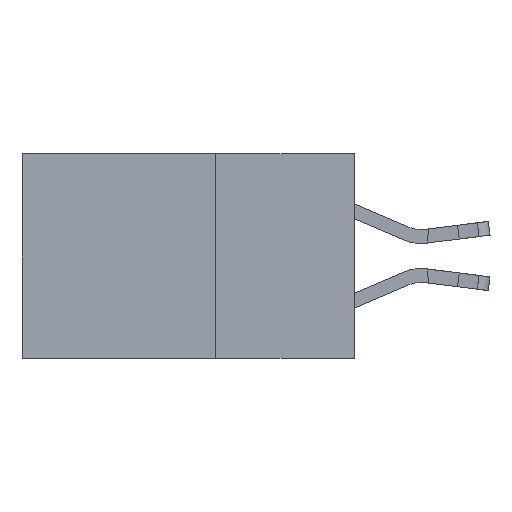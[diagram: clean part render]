
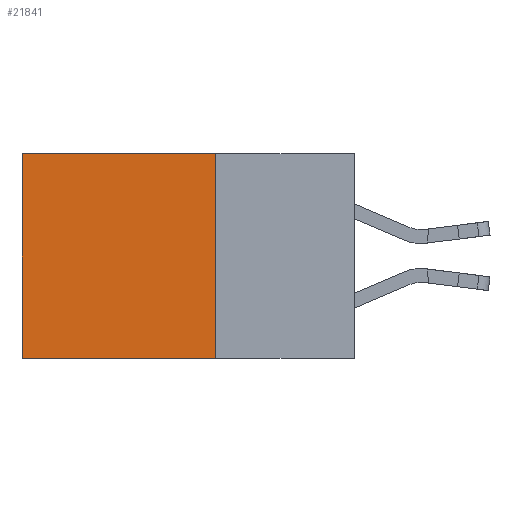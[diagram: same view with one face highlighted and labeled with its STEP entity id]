
A CAD part, left-side view. The second image highlights one B-rep face of the part: STEP entity #21841.
In plain terms, the highlighted planar face has unit normal (-1, 0, 0).
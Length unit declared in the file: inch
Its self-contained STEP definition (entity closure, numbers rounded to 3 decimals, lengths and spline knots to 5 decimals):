
#65 = LINE ( 'NONE', #18671, #18325 ) ;
#233 = LINE ( 'NONE', #8645, #21124 ) ;
#1150 = CARTESIAN_POINT ( 'NONE',  ( 0.2615, 0.25, 0. ) ) ;
#2202 = DIRECTION ( 'NONE',  ( 0., 0., -1. ) ) ;
#2659 = CARTESIAN_POINT ( 'NONE',  ( 0.2615, 0.6, -0.37 ) ) ;
#3475 = EDGE_CURVE ( 'NONE', #10240, #20076, #233, .T. ) ;
#3561 = ORIENTED_EDGE ( 'NONE', *, *, #3475, .F. ) ;
#3818 = VERTEX_POINT ( 'NONE', #10175 ) ;
#3977 = EDGE_CURVE ( 'NONE', #10240, #3818, #4320, .T. ) ;
#4320 = LINE ( 'NONE', #1150, #20062 ) ;
#6410 = DIRECTION ( 'NONE',  ( 1., 0., 0. ) ) ;
#7657 = AXIS2_PLACEMENT_3D ( 'NONE', #21619, #6410, #19941 ) ;
#8099 = FACE_OUTER_BOUND ( 'NONE', #13584, .T. ) ;
#8645 = CARTESIAN_POINT ( 'NONE',  ( 0.2615, 0.25, -0.37 ) ) ;
#9176 = ORIENTED_EDGE ( 'NONE', *, *, #10137, .F. ) ;
#9628 = ORIENTED_EDGE ( 'NONE', *, *, #3977, .T. ) ;
#10137 = EDGE_CURVE ( 'NONE', #20076, #20198, #65, .T. ) ;
#10175 = CARTESIAN_POINT ( 'NONE',  ( 0.2615, 0.6, 0. ) ) ;
#10240 = VERTEX_POINT ( 'NONE', #15453 ) ;
#10302 = ORIENTED_EDGE ( 'NONE', *, *, #20506, .T. ) ;
#12171 = CARTESIAN_POINT ( 'NONE',  ( 0.2615, 0.6, -0.37 ) ) ;
#13584 = EDGE_LOOP ( 'NONE', ( #10302, #9176, #3561, #9628 ) ) ;
#13974 = CARTESIAN_POINT ( 'NONE',  ( 0.2615, 0.25, -0.37 ) ) ;
#14558 = DIRECTION ( 'NONE',  ( 0., 1., 0. ) ) ;
#14868 = PLANE ( 'NONE',  #7657 ) ;
#15412 = DIRECTION ( 'NONE',  ( 0., 0., -1. ) ) ;
#15453 = CARTESIAN_POINT ( 'NONE',  ( 0.2615, 0.25, 0. ) ) ;
#16698 = DIRECTION ( 'NONE',  ( 0., 1., 0. ) ) ;
#17503 = VECTOR ( 'NONE', #2202, 39.37008 ) ;
#18325 = VECTOR ( 'NONE', #16698, 39.37008 ) ;
#18671 = CARTESIAN_POINT ( 'NONE',  ( 0.2615, 0.25, -0.37 ) ) ;
#18724 = LINE ( 'NONE', #12171, #17503 ) ;
#19941 = DIRECTION ( 'NONE',  ( 0., 0., -1. ) ) ;
#20062 = VECTOR ( 'NONE', #14558, 39.37008 ) ;
#20076 = VERTEX_POINT ( 'NONE', #13974 ) ;
#20198 = VERTEX_POINT ( 'NONE', #2659 ) ;
#20506 = EDGE_CURVE ( 'NONE', #3818, #20198, #18724, .T. ) ;
#21124 = VECTOR ( 'NONE', #15412, 39.37008 ) ;
#21619 = CARTESIAN_POINT ( 'NONE',  ( 0.2615, 0.25, -0.37 ) ) ;
#21841 = ADVANCED_FACE ( 'NONE', ( #8099 ), #14868, .F. ) ;
